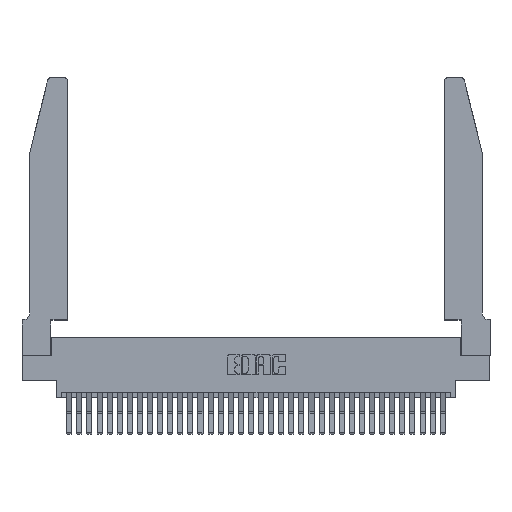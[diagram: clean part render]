
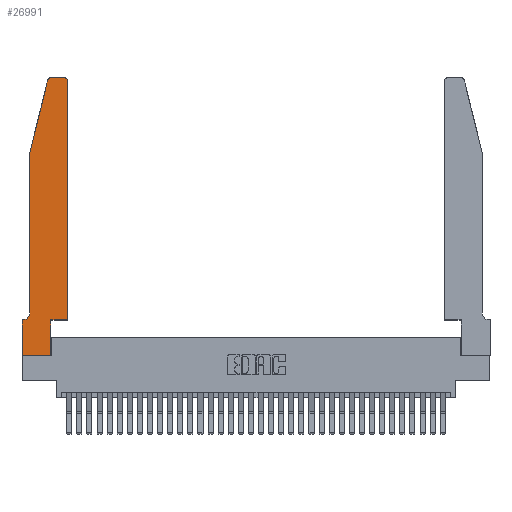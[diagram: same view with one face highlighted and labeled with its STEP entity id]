
A CAD part, top view. The second image highlights one B-rep face of the part: STEP entity #26991.
In plain terms, the highlighted planar face has unit normal (0, 0, 1).
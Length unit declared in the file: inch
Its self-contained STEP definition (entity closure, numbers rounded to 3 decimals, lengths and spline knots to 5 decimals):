
#638 = CARTESIAN_POINT ( 'NONE',  ( 0.2865, 0., 0.37 ) ) ;
#909 = ORIENTED_EDGE ( 'NONE', *, *, #12237, .T. ) ;
#959 = ORIENTED_EDGE ( 'NONE', *, *, #4228, .T. ) ;
#1642 = CARTESIAN_POINT ( 'NONE',  ( 0.284, 2.72, 0.37 ) ) ;
#1936 = DIRECTION ( 'NONE',  ( 1., 0., 0. ) ) ;
#2097 = ORIENTED_EDGE ( 'NONE', *, *, #4167, .T. ) ;
#2377 = VERTEX_POINT ( 'NONE', #32227 ) ;
#3003 = EDGE_CURVE ( 'NONE', #4446, #5542, #18699, .T. ) ;
#3132 = ORIENTED_EDGE ( 'NONE', *, *, #7636, .T. ) ;
#3375 = VECTOR ( 'NONE', #9907, 39.37008 ) ;
#3470 = VECTOR ( 'NONE', #25264, 39.37008 ) ;
#3692 = ORIENTED_EDGE ( 'NONE', *, *, #3003, .T. ) ;
#3799 = CARTESIAN_POINT ( 'NONE',  ( 0., 0., 0.37 ) ) ;
#4167 = EDGE_CURVE ( 'NONE', #7360, #34157, #22545, .T. ) ;
#4218 = LINE ( 'NONE', #27850, #10675 ) ;
#4228 = EDGE_CURVE ( 'NONE', #9281, #23359, #13602, .T. ) ;
#4446 = VERTEX_POINT ( 'NONE', #17069 ) ;
#4735 = CARTESIAN_POINT ( 'NONE',  ( 0.4205, 2.72, 0.37 ) ) ;
#4932 = PLANE ( 'NONE',  #24200 ) ;
#5542 = VERTEX_POINT ( 'NONE', #3799 ) ;
#6248 = LINE ( 'NONE', #33990, #34476 ) ;
#6705 = DIRECTION ( 'NONE',  ( 0., -1., 0. ) ) ;
#6750 = EDGE_CURVE ( 'NONE', #22951, #2377, #21579, .T. ) ;
#7006 = ORIENTED_EDGE ( 'NONE', *, *, #21103, .T. ) ;
#7135 = DIRECTION ( 'NONE',  ( 1., 0., 0. ) ) ;
#7360 = VERTEX_POINT ( 'NONE', #15488 ) ;
#7434 = CARTESIAN_POINT ( 'NONE',  ( 0.4505, 0.35, 0.37 ) ) ;
#7496 = EDGE_LOOP ( 'NONE', ( #2097, #909, #19720, #3132, #959, #10628, #3692, #30517, #12186, #20750, #7006, #12366 ) ) ;
#7636 = EDGE_CURVE ( 'NONE', #24242, #9281, #14631, .T. ) ;
#8648 = AXIS2_PLACEMENT_3D ( 'NONE', #4735, #26497, #14596 ) ;
#8890 = CARTESIAN_POINT ( 'NONE',  ( 0.2865, 0.35, 0.37 ) ) ;
#9115 = CARTESIAN_POINT ( 'NONE',  ( 0.0755, 0.42, 0.37 ) ) ;
#9281 = VERTEX_POINT ( 'NONE', #9115 ) ;
#9907 = DIRECTION ( 'NONE',  ( 0., 1., 0. ) ) ;
#10147 = VERTEX_POINT ( 'NONE', #20169 ) ;
#10230 = EDGE_CURVE ( 'NONE', #5542, #14925, #6248, .T. ) ;
#10628 = ORIENTED_EDGE ( 'NONE', *, *, #16874, .T. ) ;
#10630 = DIRECTION ( 'NONE',  ( 0., 0., -1. ) ) ;
#10675 = VECTOR ( 'NONE', #14512, 39.37008 ) ;
#10932 = CARTESIAN_POINT ( 'NONE',  ( 0.0055, 0.35, 0.37 ) ) ;
#11335 = VECTOR ( 'NONE', #15662, 39.37008 ) ;
#12186 = ORIENTED_EDGE ( 'NONE', *, *, #19826, .T. ) ;
#12237 = EDGE_CURVE ( 'NONE', #34157, #10147, #28814, .T. ) ;
#12366 = ORIENTED_EDGE ( 'NONE', *, *, #18820, .T. ) ;
#12509 = LINE ( 'NONE', #8890, #3470 ) ;
#12533 = CARTESIAN_POINT ( 'NONE',  ( 0.4505, 0.35, 0.37 ) ) ;
#12723 = CARTESIAN_POINT ( 'NONE',  ( 0.4505, 2.72, 0.37 ) ) ;
#13602 = CIRCLE ( 'NONE', #27408, 0.07 ) ;
#14341 = LINE ( 'NONE', #27490, #26295 ) ;
#14512 = DIRECTION ( 'NONE',  ( -0.239, -0.971, 0. ) ) ;
#14596 = DIRECTION ( 'NONE',  ( 1., 0., 0. ) ) ;
#14631 = LINE ( 'NONE', #25833, #21522 ) ;
#14925 = VERTEX_POINT ( 'NONE', #638 ) ;
#15488 = CARTESIAN_POINT ( 'NONE',  ( 0.4205, 2.75, 0.37 ) ) ;
#15662 = DIRECTION ( 'NONE',  ( 0., -1., 0. ) ) ;
#15812 = EDGE_CURVE ( 'NONE', #10147, #24242, #4218, .T. ) ;
#16024 = CARTESIAN_POINT ( 'NONE',  ( 0., 0., 0.37 ) ) ;
#16246 = DIRECTION ( 'NONE',  ( 0., 0., 1. ) ) ;
#16874 = EDGE_CURVE ( 'NONE', #23359, #4446, #14341, .T. ) ;
#17069 = CARTESIAN_POINT ( 'NONE',  ( 0., 0.35, 0.37 ) ) ;
#18699 = LINE ( 'NONE', #16024, #11335 ) ;
#18765 = VECTOR ( 'NONE', #22388, 39.37008 ) ;
#18820 = EDGE_CURVE ( 'NONE', #22864, #7360, #35176, .T. ) ;
#19199 = DIRECTION ( 'NONE',  ( 1., 0., 0. ) ) ;
#19720 = ORIENTED_EDGE ( 'NONE', *, *, #15812, .T. ) ;
#19826 = EDGE_CURVE ( 'NONE', #14925, #22951, #12509, .T. ) ;
#20169 = CARTESIAN_POINT ( 'NONE',  ( 0.25487, 2.72718, 0.37 ) ) ;
#20750 = ORIENTED_EDGE ( 'NONE', *, *, #6750, .T. ) ;
#20829 = DIRECTION ( 'NONE',  ( 0., 0., 1. ) ) ;
#21103 = EDGE_CURVE ( 'NONE', #2377, #22864, #27320, .T. ) ;
#21522 = VECTOR ( 'NONE', #6705, 39.37008 ) ;
#21579 = LINE ( 'NONE', #7434, #27876 ) ;
#22284 = DIRECTION ( 'NONE',  ( -1., 0., 0. ) ) ;
#22388 = DIRECTION ( 'NONE',  ( -1., 0., 0. ) ) ;
#22545 = LINE ( 'NONE', #26228, #18765 ) ;
#22864 = VERTEX_POINT ( 'NONE', #12723 ) ;
#22951 = VERTEX_POINT ( 'NONE', #27675 ) ;
#23359 = VERTEX_POINT ( 'NONE', #10932 ) ;
#24200 = AXIS2_PLACEMENT_3D ( 'NONE', #26697, #16246, #19199 ) ;
#24242 = VERTEX_POINT ( 'NONE', #34819 ) ;
#25264 = DIRECTION ( 'NONE',  ( 0., 1., 0. ) ) ;
#25833 = CARTESIAN_POINT ( 'NONE',  ( 0.0755, 2., 0.37 ) ) ;
#26008 = CARTESIAN_POINT ( 'NONE',  ( 0.284, 2.75, 0.37 ) ) ;
#26228 = CARTESIAN_POINT ( 'NONE',  ( 0.2605, 2.75, 0.37 ) ) ;
#26295 = VECTOR ( 'NONE', #22284, 39.37008 ) ;
#26497 = DIRECTION ( 'NONE',  ( 0., 0., 1. ) ) ;
#26697 = CARTESIAN_POINT ( 'NONE',  ( 0., 0.35, 0.37 ) ) ;
#26741 = DIRECTION ( 'NONE',  ( -1., 0., 0. ) ) ;
#26991 = ADVANCED_FACE ( 'NONE', ( #27489 ), #4932, .T. ) ;
#27320 = LINE ( 'NONE', #12533, #3375 ) ;
#27408 = AXIS2_PLACEMENT_3D ( 'NONE', #29597, #10630, #26741 ) ;
#27489 = FACE_OUTER_BOUND ( 'NONE', #7496, .T. ) ;
#27490 = CARTESIAN_POINT ( 'NONE',  ( 0.0755, 0.35, 0.37 ) ) ;
#27675 = CARTESIAN_POINT ( 'NONE',  ( 0.2865, 0.35, 0.37 ) ) ;
#27808 = AXIS2_PLACEMENT_3D ( 'NONE', #1642, #20829, #7135 ) ;
#27850 = CARTESIAN_POINT ( 'NONE',  ( 0.0755, 2., 0.37 ) ) ;
#27876 = VECTOR ( 'NONE', #1936, 39.37008 ) ;
#28814 = CIRCLE ( 'NONE', #27808, 0.03 ) ;
#29597 = CARTESIAN_POINT ( 'NONE',  ( 0.0055, 0.42, 0.37 ) ) ;
#30517 = ORIENTED_EDGE ( 'NONE', *, *, #10230, .T. ) ;
#31134 = DIRECTION ( 'NONE',  ( 1., 0., 0. ) ) ;
#32227 = CARTESIAN_POINT ( 'NONE',  ( 0.4505, 0.35, 0.37 ) ) ;
#33990 = CARTESIAN_POINT ( 'NONE',  ( 0., 0., 0.37 ) ) ;
#34157 = VERTEX_POINT ( 'NONE', #26008 ) ;
#34476 = VECTOR ( 'NONE', #31134, 39.37008 ) ;
#34819 = CARTESIAN_POINT ( 'NONE',  ( 0.0755, 2., 0.37 ) ) ;
#35176 = CIRCLE ( 'NONE', #8648, 0.03 ) ;
